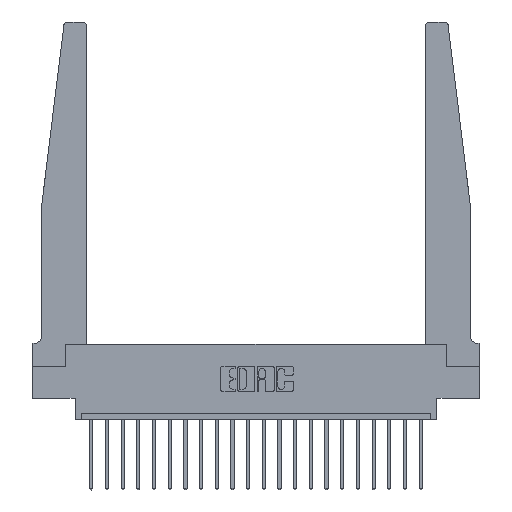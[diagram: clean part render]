
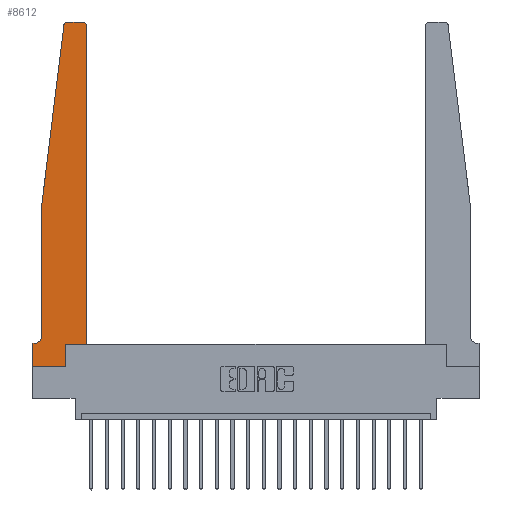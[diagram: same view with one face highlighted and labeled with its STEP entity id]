
A CAD part, top view. The second image highlights one B-rep face of the part: STEP entity #8612.
In plain terms, the highlighted planar face has unit normal (0, 0, 1).
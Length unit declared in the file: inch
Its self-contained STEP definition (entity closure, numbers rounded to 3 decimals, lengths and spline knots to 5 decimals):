
#324 = CARTESIAN_POINT ( 'NONE',  ( 0.065, 1.25, 0.37 ) ) ;
#332 = LINE ( 'NONE', #324, #10625 ) ;
#769 = CARTESIAN_POINT ( 'NONE',  ( 0., 0., 0.37 ) ) ;
#1074 = DIRECTION ( 'NONE',  ( 1., 0., 0. ) ) ;
#1247 = CARTESIAN_POINT ( 'NONE',  ( 0.25, 2.75, 0.37 ) ) ;
#2005 = ORIENTED_EDGE ( 'NONE', *, *, #20124, .T. ) ;
#2287 = LINE ( 'NONE', #20609, #15413 ) ;
#2381 = LINE ( 'NONE', #9275, #3148 ) ;
#2686 = EDGE_CURVE ( 'NONE', #5067, #4988, #19678, .T. ) ;
#2795 = CARTESIAN_POINT ( 'NONE',  ( 0.2605, 0.18, 0.37 ) ) ;
#3036 = EDGE_CURVE ( 'NONE', #8764, #7521, #17348, .T. ) ;
#3148 = VECTOR ( 'NONE', #7699, 39.37008 ) ;
#3410 = ORIENTED_EDGE ( 'NONE', *, *, #5795, .T. ) ;
#3438 = VECTOR ( 'NONE', #14472, 39.37008 ) ;
#3588 = CARTESIAN_POINT ( 'NONE',  ( 0., 0.1875, 0.37 ) ) ;
#3605 = CARTESIAN_POINT ( 'NONE',  ( 0.2605, 0.18, 0.37 ) ) ;
#3801 = DIRECTION ( 'NONE',  ( 1., 0., 0. ) ) ;
#3867 = DIRECTION ( 'NONE',  ( 0., 0., 1. ) ) ;
#4021 = CARTESIAN_POINT ( 'NONE',  ( 0.27653, 2.75, 0.37 ) ) ;
#4083 = ORIENTED_EDGE ( 'NONE', *, *, #17266, .T. ) ;
#4086 = DIRECTION ( 'NONE',  ( -0.122, -0.992, 0. ) ) ;
#4095 = VERTEX_POINT ( 'NONE', #5746 ) ;
#4256 = VECTOR ( 'NONE', #17198, 39.37008 ) ;
#4314 = DIRECTION ( 'NONE',  ( 1., 0., 0. ) ) ;
#4988 = VERTEX_POINT ( 'NONE', #8355 ) ;
#5067 = VERTEX_POINT ( 'NONE', #20322 ) ;
#5526 = EDGE_CURVE ( 'NONE', #7818, #12073, #332, .T. ) ;
#5746 = CARTESIAN_POINT ( 'NONE',  ( 0.425, 0.18, 0.37 ) ) ;
#5795 = EDGE_CURVE ( 'NONE', #18722, #16312, #8550, .T. ) ;
#5799 = ORIENTED_EDGE ( 'NONE', *, *, #3036, .T. ) ;
#5916 = ORIENTED_EDGE ( 'NONE', *, *, #5526, .T. ) ;
#5961 = CARTESIAN_POINT ( 'NONE',  ( 0.27653, 2.72, 0.37 ) ) ;
#6336 = CARTESIAN_POINT ( 'NONE',  ( 0.2605, 0., 0.37 ) ) ;
#6445 = CARTESIAN_POINT ( 'NONE',  ( 0.395, 2.75, 0.37 ) ) ;
#6838 = LINE ( 'NONE', #14306, #10706 ) ;
#7039 = VECTOR ( 'NONE', #21112, 39.37008 ) ;
#7059 = ORIENTED_EDGE ( 'NONE', *, *, #11237, .T. ) ;
#7155 = CARTESIAN_POINT ( 'NONE',  ( 0.015, 0.1875, 0.37 ) ) ;
#7157 = CARTESIAN_POINT ( 'NONE',  ( 0.425, 0.18, 0.37 ) ) ;
#7521 = VERTEX_POINT ( 'NONE', #13511 ) ;
#7671 = ORIENTED_EDGE ( 'NONE', *, *, #16695, .T. ) ;
#7698 = DIRECTION ( 'NONE',  ( 1., 0., 0. ) ) ;
#7699 = DIRECTION ( 'NONE',  ( -1., 0., 0. ) ) ;
#7763 = CIRCLE ( 'NONE', #19742, 0.05 ) ;
#7818 = VERTEX_POINT ( 'NONE', #14453 ) ;
#7859 = LINE ( 'NONE', #14179, #16560 ) ;
#7888 = AXIS2_PLACEMENT_3D ( 'NONE', #14373, #12569, #7698 ) ;
#8355 = CARTESIAN_POINT ( 'NONE',  ( 0., 0., 0.37 ) ) ;
#8375 = ORIENTED_EDGE ( 'NONE', *, *, #14481, .T. ) ;
#8550 = CIRCLE ( 'NONE', #7888, 0.03 ) ;
#8559 = PLANE ( 'NONE',  #12722 ) ;
#8612 = ADVANCED_FACE ( 'NONE', ( #15356 ), #8559, .T. ) ;
#8764 = VERTEX_POINT ( 'NONE', #4021 ) ;
#9275 = CARTESIAN_POINT ( 'NONE',  ( 0.065, 0.1875, 0.37 ) ) ;
#9535 = ORIENTED_EDGE ( 'NONE', *, *, #16628, .T. ) ;
#10337 = EDGE_CURVE ( 'NONE', #12073, #15373, #7763, .T. ) ;
#10493 = ORIENTED_EDGE ( 'NONE', *, *, #2686, .T. ) ;
#10625 = VECTOR ( 'NONE', #19769, 39.37008 ) ;
#10706 = VECTOR ( 'NONE', #20960, 39.37008 ) ;
#10888 = DIRECTION ( 'NONE',  ( -1., 0., 0. ) ) ;
#11237 = EDGE_CURVE ( 'NONE', #7521, #7818, #2287, .T. ) ;
#11476 = VERTEX_POINT ( 'NONE', #6336 ) ;
#12073 = VERTEX_POINT ( 'NONE', #15174 ) ;
#12308 = DIRECTION ( 'NONE',  ( 0., 1., 0. ) ) ;
#12420 = DIRECTION ( 'NONE',  ( 0., 0., 1. ) ) ;
#12569 = DIRECTION ( 'NONE',  ( 0., 0., 1. ) ) ;
#12722 = AXIS2_PLACEMENT_3D ( 'NONE', #3588, #3867, #3801 ) ;
#12840 = VECTOR ( 'NONE', #12308, 39.37008 ) ;
#13251 = CARTESIAN_POINT ( 'NONE',  ( 0.425, 2.72, 0.37 ) ) ;
#13511 = CARTESIAN_POINT ( 'NONE',  ( 0.24675, 2.72367, 0.37 ) ) ;
#14179 = CARTESIAN_POINT ( 'NONE',  ( 0., 0., 0.37 ) ) ;
#14301 = ORIENTED_EDGE ( 'NONE', *, *, #10337, .T. ) ;
#14306 = CARTESIAN_POINT ( 'NONE',  ( 0.425, 0.18, 0.37 ) ) ;
#14373 = CARTESIAN_POINT ( 'NONE',  ( 0.395, 2.72, 0.37 ) ) ;
#14453 = CARTESIAN_POINT ( 'NONE',  ( 0.065, 1.25, 0.37 ) ) ;
#14472 = DIRECTION ( 'NONE',  ( -1., 0., 0. ) ) ;
#14481 = EDGE_CURVE ( 'NONE', #18742, #4095, #6838, .T. ) ;
#15174 = CARTESIAN_POINT ( 'NONE',  ( 0.065, 0.2375, 0.37 ) ) ;
#15356 = FACE_OUTER_BOUND ( 'NONE', #15862, .T. ) ;
#15373 = VERTEX_POINT ( 'NONE', #7155 ) ;
#15413 = VECTOR ( 'NONE', #4086, 39.37008 ) ;
#15689 = CARTESIAN_POINT ( 'NONE',  ( 0.015, 0.2375, 0.37 ) ) ;
#15778 = LINE ( 'NONE', #2795, #7039 ) ;
#15862 = EDGE_LOOP ( 'NONE', ( #7671, #5799, #7059, #5916, #14301, #19711, #10493, #9535, #4083, #8375, #2005, #3410 ) ) ;
#16312 = VERTEX_POINT ( 'NONE', #6445 ) ;
#16560 = VECTOR ( 'NONE', #4314, 39.37008 ) ;
#16628 = EDGE_CURVE ( 'NONE', #4988, #11476, #7859, .T. ) ;
#16695 = EDGE_CURVE ( 'NONE', #16312, #8764, #20909, .T. ) ;
#17198 = DIRECTION ( 'NONE',  ( 0., -1., 0. ) ) ;
#17266 = EDGE_CURVE ( 'NONE', #11476, #18742, #15778, .T. ) ;
#17348 = CIRCLE ( 'NONE', #21036, 0.03 ) ;
#17400 = DIRECTION ( 'NONE',  ( 0., 0., -1. ) ) ;
#18229 = EDGE_CURVE ( 'NONE', #15373, #5067, #2381, .T. ) ;
#18708 = LINE ( 'NONE', #7157, #12840 ) ;
#18722 = VERTEX_POINT ( 'NONE', #13251 ) ;
#18742 = VERTEX_POINT ( 'NONE', #3605 ) ;
#19678 = LINE ( 'NONE', #769, #4256 ) ;
#19711 = ORIENTED_EDGE ( 'NONE', *, *, #18229, .T. ) ;
#19742 = AXIS2_PLACEMENT_3D ( 'NONE', #15689, #17400, #10888 ) ;
#19769 = DIRECTION ( 'NONE',  ( 0., -1., 0. ) ) ;
#20124 = EDGE_CURVE ( 'NONE', #4095, #18722, #18708, .T. ) ;
#20322 = CARTESIAN_POINT ( 'NONE',  ( 0., 0.1875, 0.37 ) ) ;
#20609 = CARTESIAN_POINT ( 'NONE',  ( 0.065, 1.25, 0.37 ) ) ;
#20909 = LINE ( 'NONE', #1247, #3438 ) ;
#20960 = DIRECTION ( 'NONE',  ( 1., 0., 0. ) ) ;
#21036 = AXIS2_PLACEMENT_3D ( 'NONE', #5961, #12420, #1074 ) ;
#21112 = DIRECTION ( 'NONE',  ( 0., 1., 0. ) ) ;
